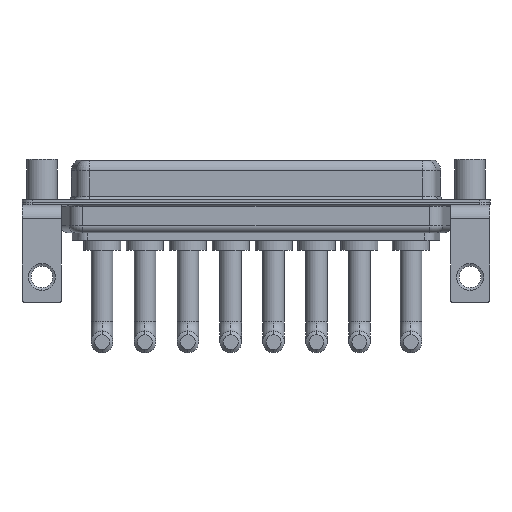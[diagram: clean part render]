
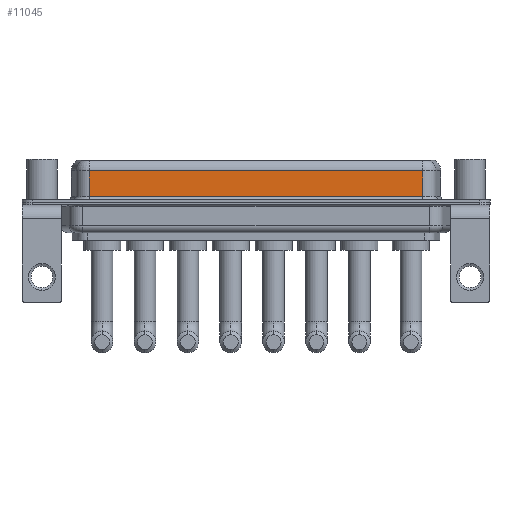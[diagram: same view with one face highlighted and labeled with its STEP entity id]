
A CAD part, front view. The second image highlights one B-rep face of the part: STEP entity #11045.
In plain terms, the highlighted planar face has unit normal (0, -1, 0).
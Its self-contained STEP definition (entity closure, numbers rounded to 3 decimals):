
#371 = VERTEX_POINT ( 'NONE', #2617 ) ;
#656 = VERTEX_POINT ( 'NONE', #14459 ) ;
#664 = LINE ( 'NONE', #15317, #7546 ) ;
#970 = DIRECTION ( 'NONE',  ( -1., 0., 0. ) ) ;
#974 = EDGE_CURVE ( 'NONE', #8694, #656, #664, .T. ) ;
#1726 = DIRECTION ( 'NONE',  ( 0., 0., 1. ) ) ;
#2188 = CARTESIAN_POINT ( 'NONE',  ( 56.462, -3.95, 6.4 ) ) ;
#2271 = ORIENTED_EDGE ( 'NONE', *, *, #7721, .T. ) ;
#2352 = CARTESIAN_POINT ( 'NONE',  ( 56.462, -3.95, 0.9 ) ) ;
#2617 = CARTESIAN_POINT ( 'NONE',  ( 56.462, -3.95, 0.9 ) ) ;
#3128 = ORIENTED_EDGE ( 'NONE', *, *, #974, .T. ) ;
#3668 = LINE ( 'NONE', #14647, #5826 ) ;
#4460 = CARTESIAN_POINT ( 'NONE',  ( 7.038, -3.95, 0.9 ) ) ;
#5409 = ORIENTED_EDGE ( 'NONE', *, *, #10950, .F. ) ;
#5777 = EDGE_LOOP ( 'NONE', ( #5409, #3128, #2271, #7617 ) ) ;
#5826 = VECTOR ( 'NONE', #6253, 1000. ) ;
#6253 = DIRECTION ( 'NONE',  ( 0., 0., -1. ) ) ;
#6343 = EDGE_CURVE ( 'NONE', #12377, #371, #14681, .T. ) ;
#7546 = VECTOR ( 'NONE', #970, 1000. ) ;
#7617 = ORIENTED_EDGE ( 'NONE', *, *, #6343, .T. ) ;
#7721 = EDGE_CURVE ( 'NONE', #656, #12377, #3668, .T. ) ;
#8694 = VERTEX_POINT ( 'NONE', #10905 ) ;
#9473 = DIRECTION ( 'NONE',  ( 0., 0., -1. ) ) ;
#9714 = DIRECTION ( 'NONE',  ( 1., 0., 0. ) ) ;
#10288 = CARTESIAN_POINT ( 'NONE',  ( 56.462, -3.95, 6.4 ) ) ;
#10747 = DIRECTION ( 'NONE',  ( 0., 1., 0. ) ) ;
#10905 = CARTESIAN_POINT ( 'NONE',  ( 56.462, -3.95, 4.65 ) ) ;
#10950 = EDGE_CURVE ( 'NONE', #8694, #371, #11481, .T. ) ;
#11045 = ADVANCED_FACE ( 'NONE', ( #12786 ), #13165, .F. ) ;
#11481 = LINE ( 'NONE', #10288, #15611 ) ;
#12377 = VERTEX_POINT ( 'NONE', #4460 ) ;
#12786 = FACE_OUTER_BOUND ( 'NONE', #5777, .T. ) ;
#13165 = PLANE ( 'NONE',  #14100 ) ;
#14100 = AXIS2_PLACEMENT_3D ( 'NONE', #2188, #10747, #1726 ) ;
#14459 = CARTESIAN_POINT ( 'NONE',  ( 7.038, -3.95, 4.65 ) ) ;
#14647 = CARTESIAN_POINT ( 'NONE',  ( 7.038, -3.95, 6.4 ) ) ;
#14681 = LINE ( 'NONE', #2352, #14734 ) ;
#14734 = VECTOR ( 'NONE', #9714, 1000. ) ;
#15317 = CARTESIAN_POINT ( 'NONE',  ( 56.462, -3.95, 4.65 ) ) ;
#15611 = VECTOR ( 'NONE', #9473, 1000. ) ;
